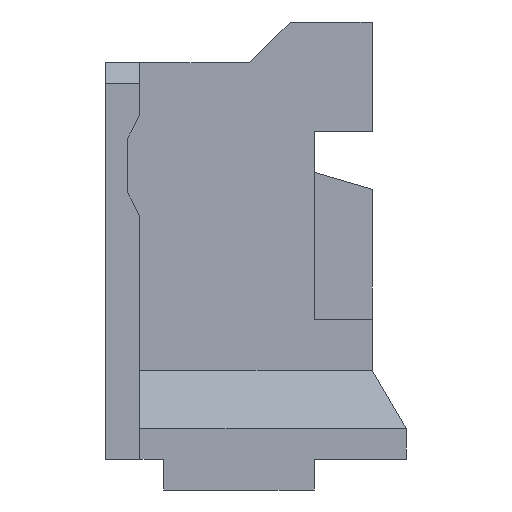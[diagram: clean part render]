
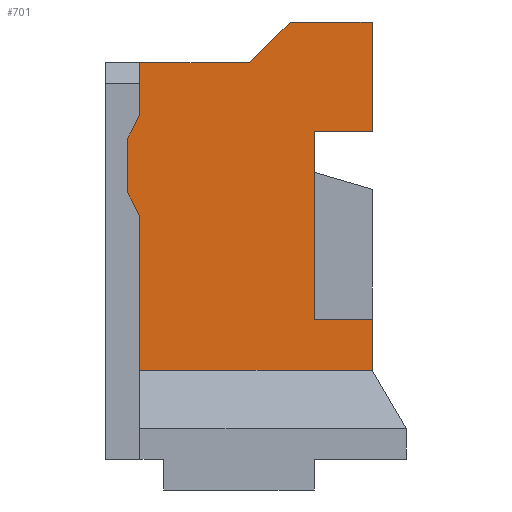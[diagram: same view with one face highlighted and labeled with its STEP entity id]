
A CAD part, left-side view. The second image highlights one B-rep face of the part: STEP entity #701.
In plain terms, the highlighted planar face has unit normal (-1, 0, 0).
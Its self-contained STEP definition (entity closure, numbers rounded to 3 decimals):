
#36 = LINE ( 'NONE', #6242, #6473 ) ;
#262 = ORIENTED_EDGE ( 'NONE', *, *, #4194, .F. ) ;
#325 = EDGE_CURVE ( 'NONE', #9602, #4634, #6915, .T. ) ;
#328 = DIRECTION ( 'NONE',  ( 0., 0., -1. ) ) ;
#431 = VECTOR ( 'NONE', #7724, 1000. ) ;
#465 = CARTESIAN_POINT ( 'NONE',  ( -1.25, -1.45, -3.75 ) ) ;
#559 = CARTESIAN_POINT ( 'NONE',  ( -1.25, -1.1, 0.6 ) ) ;
#656 = VERTEX_POINT ( 'NONE', #3108 ) ;
#701 = ADVANCED_FACE ( 'NONE', ( #4017 ), #4711, .F. ) ;
#721 = CARTESIAN_POINT ( 'NONE',  ( -1.25, 1.1, -4.5 ) ) ;
#761 = AXIS2_PLACEMENT_3D ( 'NONE', #8421, #1683, #2527 ) ;
#853 = VERTEX_POINT ( 'NONE', #1822 ) ;
#955 = ORIENTED_EDGE ( 'NONE', *, *, #4812, .F. ) ;
#1086 = ORIENTED_EDGE ( 'NONE', *, *, #6917, .F. ) ;
#1096 = VERTEX_POINT ( 'NONE', #4864 ) ;
#1235 = DIRECTION ( 'NONE',  ( 0., 0., -1. ) ) ;
#1403 = EDGE_CURVE ( 'NONE', #7521, #1096, #8841, .T. ) ;
#1493 = DIRECTION ( 'NONE',  ( 0., 0.447, 0.894 ) ) ;
#1683 = DIRECTION ( 'NONE',  ( 1., 0., 0. ) ) ;
#1822 = CARTESIAN_POINT ( 'NONE',  ( -1.25, -1.45, -1. ) ) ;
#2034 = VECTOR ( 'NONE', #5505, 1000. ) ;
#2035 = CARTESIAN_POINT ( 'NONE',  ( -1.25, -1.45, -1. ) ) ;
#2180 = VECTOR ( 'NONE', #328, 1000. ) ;
#2343 = ORIENTED_EDGE ( 'NONE', *, *, #8941, .F. ) ;
#2344 = CARTESIAN_POINT ( 'NONE',  ( -1.25, 1.275, -1.9 ) ) ;
#2373 = VECTOR ( 'NONE', #9103, 1000. ) ;
#2527 = DIRECTION ( 'NONE',  ( 0., 0., -1. ) ) ;
#2647 = DIRECTION ( 'NONE',  ( 0., 0., 1. ) ) ;
#2858 = EDGE_CURVE ( 'NONE', #3533, #6128, #8924, .T. ) ;
#3108 = CARTESIAN_POINT ( 'NONE',  ( -1.25, 1.1, 0. ) ) ;
#3301 = ORIENTED_EDGE ( 'NONE', *, *, #6676, .F. ) ;
#3387 = DIRECTION ( 'NONE',  ( 0., -1., 0. ) ) ;
#3393 = CARTESIAN_POINT ( 'NONE',  ( -1.25, 1.1, -5.8 ) ) ;
#3458 = LINE ( 'NONE', #559, #2373 ) ;
#3531 = CARTESIAN_POINT ( 'NONE',  ( -1.25, -2.3, -1. ) ) ;
#3533 = VERTEX_POINT ( 'NONE', #7246 ) ;
#3564 = DIRECTION ( 'NONE',  ( 0., 1., 0. ) ) ;
#3634 = CARTESIAN_POINT ( 'NONE',  ( -1.25, -0.5, 0. ) ) ;
#3642 = CARTESIAN_POINT ( 'NONE',  ( -1.25, -1.1, 0.6 ) ) ;
#3808 = VERTEX_POINT ( 'NONE', #3634 ) ;
#3838 = VERTEX_POINT ( 'NONE', #465 ) ;
#4017 = FACE_OUTER_BOUND ( 'NONE', #4862, .T. ) ;
#4163 = LINE ( 'NONE', #3531, #8045 ) ;
#4178 = LINE ( 'NONE', #2035, #7563 ) ;
#4190 = LINE ( 'NONE', #5657, #8411 ) ;
#4194 = EDGE_CURVE ( 'NONE', #6128, #9602, #6844, .T. ) ;
#4298 = ORIENTED_EDGE ( 'NONE', *, *, #5356, .F. ) ;
#4634 = VERTEX_POINT ( 'NONE', #9839 ) ;
#4711 = PLANE ( 'NONE',  #761 ) ;
#4801 = ORIENTED_EDGE ( 'NONE', *, *, #9376, .F. ) ;
#4812 = EDGE_CURVE ( 'NONE', #4634, #7404, #36, .T. ) ;
#4862 = EDGE_LOOP ( 'NONE', ( #9830, #4298, #3301, #955, #7806, #262, #7996, #8168, #4801, #5162, #6714, #8465, #2343, #1086 ) ) ;
#4864 = CARTESIAN_POINT ( 'NONE',  ( -1.25, -2.3, -1. ) ) ;
#5105 = EDGE_CURVE ( 'NONE', #1096, #853, #4163, .T. ) ;
#5159 = DIRECTION ( 'NONE',  ( 0., -0.707, 0.707 ) ) ;
#5162 = ORIENTED_EDGE ( 'NONE', *, *, #5105, .F. ) ;
#5356 = EDGE_CURVE ( 'NONE', #9366, #9934, #8784, .T. ) ;
#5505 = DIRECTION ( 'NONE',  ( 0., -1., 0. ) ) ;
#5506 = VERTEX_POINT ( 'NONE', #3642 ) ;
#5518 = VECTOR ( 'NONE', #9850, 1000. ) ;
#5530 = VECTOR ( 'NONE', #5159, 1000. ) ;
#5564 = LINE ( 'NONE', #7689, #8933 ) ;
#5657 = CARTESIAN_POINT ( 'NONE',  ( -1.25, 1.1, -5.8 ) ) ;
#6021 = CARTESIAN_POINT ( 'NONE',  ( -1.25, -2.3, -4.5 ) ) ;
#6128 = VERTEX_POINT ( 'NONE', #6021 ) ;
#6225 = CARTESIAN_POINT ( 'NONE',  ( -1.25, -2.3, 0.6 ) ) ;
#6242 = CARTESIAN_POINT ( 'NONE',  ( -1.25, 1.1, -2.25 ) ) ;
#6429 = CARTESIAN_POINT ( 'NONE',  ( -1.25, 3.057, -3.75 ) ) ;
#6464 = DIRECTION ( 'NONE',  ( 0., 0., 1. ) ) ;
#6473 = VECTOR ( 'NONE', #1493, 1000. ) ;
#6481 = VECTOR ( 'NONE', #8695, 1000. ) ;
#6676 = EDGE_CURVE ( 'NONE', #7404, #9366, #5564, .T. ) ;
#6693 = CARTESIAN_POINT ( 'NONE',  ( -1.25, 1.1, -0.75 ) ) ;
#6714 = ORIENTED_EDGE ( 'NONE', *, *, #1403, .F. ) ;
#6738 = VECTOR ( 'NONE', #3387, 1000. ) ;
#6844 = LINE ( 'NONE', #8588, #6481 ) ;
#6915 = LINE ( 'NONE', #3393, #8969 ) ;
#6917 = EDGE_CURVE ( 'NONE', #656, #3808, #9426, .T. ) ;
#7041 = CARTESIAN_POINT ( 'NONE',  ( -1.25, -2.3, -1.85 ) ) ;
#7246 = CARTESIAN_POINT ( 'NONE',  ( -1.25, -2.3, -3.75 ) ) ;
#7404 = VERTEX_POINT ( 'NONE', #2344 ) ;
#7521 = VERTEX_POINT ( 'NONE', #6225 ) ;
#7563 = VECTOR ( 'NONE', #1235, 1000. ) ;
#7669 = EDGE_CURVE ( 'NONE', #3838, #3533, #9769, .T. ) ;
#7689 = CARTESIAN_POINT ( 'NONE',  ( -1.25, 1.275, -2.25 ) ) ;
#7724 = DIRECTION ( 'NONE',  ( 0., 0., -1. ) ) ;
#7806 = ORIENTED_EDGE ( 'NONE', *, *, #325, .F. ) ;
#7996 = ORIENTED_EDGE ( 'NONE', *, *, #2858, .F. ) ;
#8045 = VECTOR ( 'NONE', #3564, 1000. ) ;
#8168 = ORIENTED_EDGE ( 'NONE', *, *, #7669, .F. ) ;
#8411 = VECTOR ( 'NONE', #6464, 1000. ) ;
#8421 = CARTESIAN_POINT ( 'NONE',  ( -1.25, 0., 0. ) ) ;
#8465 = ORIENTED_EDGE ( 'NONE', *, *, #9004, .F. ) ;
#8574 = CARTESIAN_POINT ( 'NONE',  ( -1.25, 1.1, 0. ) ) ;
#8588 = CARTESIAN_POINT ( 'NONE',  ( -1.25, -3., -4.5 ) ) ;
#8695 = DIRECTION ( 'NONE',  ( 0., 1., 0. ) ) ;
#8784 = LINE ( 'NONE', #6693, #5518 ) ;
#8841 = LINE ( 'NONE', #9629, #2180 ) ;
#8924 = LINE ( 'NONE', #7041, #431 ) ;
#8928 = CARTESIAN_POINT ( 'NONE',  ( -1.25, -0.5, 0. ) ) ;
#8933 = VECTOR ( 'NONE', #9916, 1000. ) ;
#8941 = EDGE_CURVE ( 'NONE', #3808, #5506, #9644, .T. ) ;
#8969 = VECTOR ( 'NONE', #2647, 1000. ) ;
#8993 = CARTESIAN_POINT ( 'NONE',  ( -1.25, 1.275, -1.1 ) ) ;
#9004 = EDGE_CURVE ( 'NONE', #5506, #7521, #3458, .T. ) ;
#9103 = DIRECTION ( 'NONE',  ( 0., -1., 0. ) ) ;
#9242 = EDGE_CURVE ( 'NONE', #9934, #656, #4190, .T. ) ;
#9366 = VERTEX_POINT ( 'NONE', #8993 ) ;
#9376 = EDGE_CURVE ( 'NONE', #853, #3838, #4178, .T. ) ;
#9426 = LINE ( 'NONE', #8574, #2034 ) ;
#9602 = VERTEX_POINT ( 'NONE', #721 ) ;
#9629 = CARTESIAN_POINT ( 'NONE',  ( -1.25, -2.3, 0.6 ) ) ;
#9644 = LINE ( 'NONE', #8928, #5530 ) ;
#9769 = LINE ( 'NONE', #6429, #6738 ) ;
#9830 = ORIENTED_EDGE ( 'NONE', *, *, #9242, .F. ) ;
#9839 = CARTESIAN_POINT ( 'NONE',  ( -1.25, 1.1, -2.25 ) ) ;
#9850 = DIRECTION ( 'NONE',  ( 0., -0.447, 0.894 ) ) ;
#9916 = DIRECTION ( 'NONE',  ( 0., 0., 1. ) ) ;
#9934 = VERTEX_POINT ( 'NONE', #9941 ) ;
#9941 = CARTESIAN_POINT ( 'NONE',  ( -1.25, 1.1, -0.75 ) ) ;
